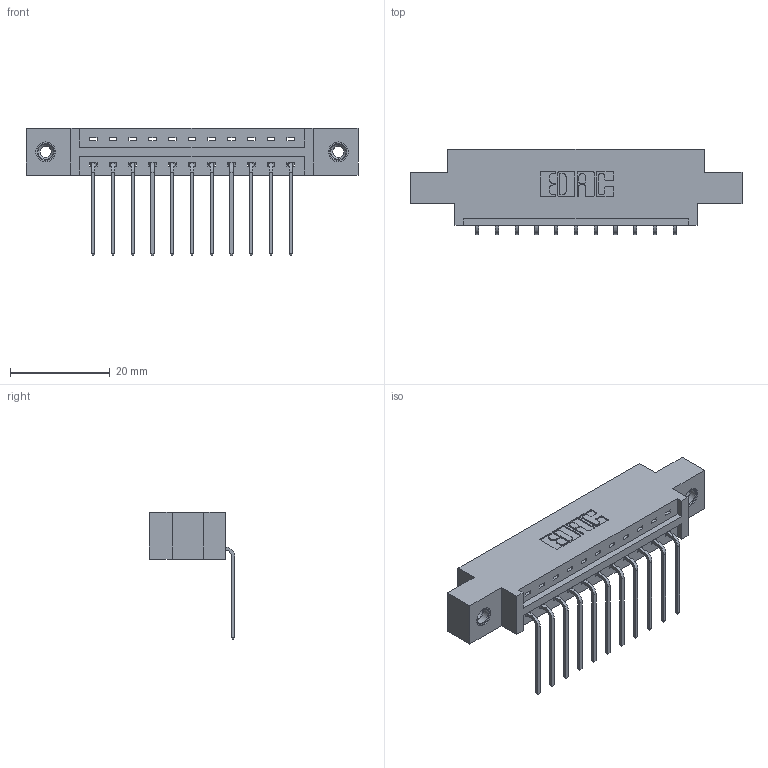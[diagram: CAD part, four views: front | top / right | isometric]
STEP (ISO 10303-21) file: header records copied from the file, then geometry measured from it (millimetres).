
FILE_DESCRIPTION (( 'STEP AP203' ), '1' );
FILE_NAME ('387-011-559-608.STEP', '2018-09-10T09:13:38', ( '' ), ( '' ), 'SwSTEP 2.0', 'SolidWorks 2016', '' );
FILE_SCHEMA (( 'CONFIG_CONTROL_DESIGN' ));
Length unit declared in the file: inch
Products named in the file (4): 337 Part_0.170 Offset - 0.156 Dia-TI; 345-292-001_558 559 Tail - 1; 345-250-001_345-250-003-102; 387-011-559-608
Assembly tree (14 placements, depth 2):
  387-011-559-608
    337 Part_0.170 Offset - 0.156 Dia-TI
    345-292-001_558 559 Tail - 1  x11
    345-250-001_345-250-003-102  x2
Bounding box: 66.6 x 17.09 x 25.53 mm (x, y, z)
Volume: 6446.5 mm3; surface area: 6840.8 mm2
Topology: 14 solids, 14 shells, 882 faces, 2593 edges, 1706 vertices
Faces by surface type: plane 634, cylinder 232, cone 12, torus 4
Entity records: 13588 total; most frequent: CARTESIAN_POINT 2346, ORIENTED_EDGE 2286, DIRECTION 2071, EDGE_CURVE 1143, VECTOR 995, LINE 995, VERTEX_POINT 756, AXIS2_PLACEMENT_3D 538
